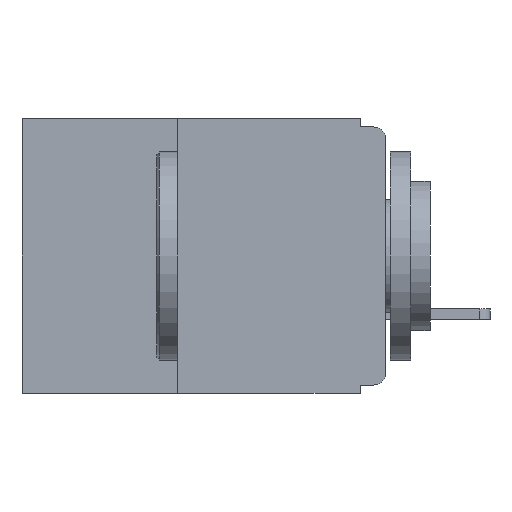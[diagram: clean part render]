
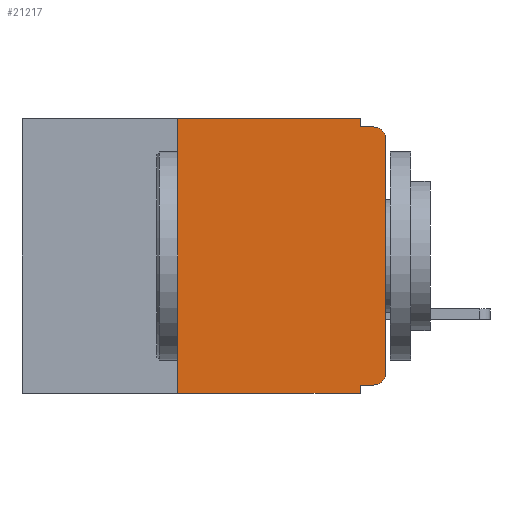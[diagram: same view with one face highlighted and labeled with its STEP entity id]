
A CAD part, left-side view. The second image highlights one B-rep face of the part: STEP entity #21217.
In plain terms, the highlighted planar face has unit normal (-1, 0, 0).
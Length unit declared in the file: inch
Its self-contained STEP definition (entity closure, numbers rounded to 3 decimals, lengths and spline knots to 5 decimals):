
#76 = ORIENTED_EDGE ( 'NONE', *, *, #14509, .T. ) ;
#262 = VERTEX_POINT ( 'NONE', #20930 ) ;
#1431 = ORIENTED_EDGE ( 'NONE', *, *, #22499, .F. ) ;
#1726 = LINE ( 'NONE', #13594, #11284 ) ;
#1873 = CARTESIAN_POINT ( 'NONE',  ( 0., 0.031, 0. ) ) ;
#2783 = CARTESIAN_POINT ( 'NONE',  ( 0., 0.031, -0.33 ) ) ;
#2972 = VERTEX_POINT ( 'NONE', #15568 ) ;
#3014 = DIRECTION ( 'NONE',  ( 1., 0., 0. ) ) ;
#3465 = CARTESIAN_POINT ( 'NONE',  ( 0., 0.437, 0. ) ) ;
#3962 = VERTEX_POINT ( 'NONE', #11965 ) ;
#4396 = DIRECTION ( 'NONE',  ( 0., 0., 1. ) ) ;
#4666 = VERTEX_POINT ( 'NONE', #12982 ) ;
#4954 = AXIS2_PLACEMENT_3D ( 'NONE', #10479, #23511, #12380 ) ;
#4986 = EDGE_CURVE ( 'NONE', #5842, #9001, #12951, .T. ) ;
#5301 = EDGE_CURVE ( 'NONE', #12902, #4666, #10860, .T. ) ;
#5350 = DIRECTION ( 'NONE',  ( 0., -1., 0. ) ) ;
#5389 = DIRECTION ( 'NONE',  ( 0., -1., 0. ) ) ;
#5541 = CARTESIAN_POINT ( 'NONE',  ( 0., 0.015, -0.305 ) ) ;
#5785 = VECTOR ( 'NONE', #5389, 39.37008 ) ;
#5842 = VERTEX_POINT ( 'NONE', #23869 ) ;
#6210 = EDGE_CURVE ( 'NONE', #6673, #262, #18990, .T. ) ;
#6287 = VECTOR ( 'NONE', #7058, 39.37008 ) ;
#6673 = VERTEX_POINT ( 'NONE', #7911 ) ;
#7019 = EDGE_CURVE ( 'NONE', #2972, #262, #21287, .T. ) ;
#7058 = DIRECTION ( 'NONE',  ( 0., -1., 0. ) ) ;
#7256 = CARTESIAN_POINT ( 'NONE',  ( 0., 0.031, 0. ) ) ;
#7468 = DIRECTION ( 'NONE',  ( 0., 0., -1. ) ) ;
#7911 = CARTESIAN_POINT ( 'NONE',  ( 0., 0.031, -0.32 ) ) ;
#8076 = CARTESIAN_POINT ( 'NONE',  ( 0., 0.015, -0.32 ) ) ;
#8418 = ORIENTED_EDGE ( 'NONE', *, *, #13133, .F. ) ;
#8632 = LINE ( 'NONE', #3465, #13662 ) ;
#9001 = VERTEX_POINT ( 'NONE', #12977 ) ;
#9172 = DIRECTION ( 'NONE',  ( 0., 0., -1. ) ) ;
#9585 = CIRCLE ( 'NONE', #4954, 0.015 ) ;
#9639 = VECTOR ( 'NONE', #16034, 39.37008 ) ;
#9664 = EDGE_CURVE ( 'NONE', #14333, #5842, #16565, .T. ) ;
#9904 = VECTOR ( 'NONE', #10613, 39.37008 ) ;
#10479 = CARTESIAN_POINT ( 'NONE',  ( 0., 0.015, -0.025 ) ) ;
#10613 = DIRECTION ( 'NONE',  ( 0., 1., 0. ) ) ;
#10860 = LINE ( 'NONE', #12954, #5785 ) ;
#11175 = ORIENTED_EDGE ( 'NONE', *, *, #6210, .F. ) ;
#11284 = VECTOR ( 'NONE', #13673, 39.37008 ) ;
#11965 = CARTESIAN_POINT ( 'NONE',  ( 0., 0.25, 0. ) ) ;
#12380 = DIRECTION ( 'NONE',  ( 0., 0., -1. ) ) ;
#12902 = VERTEX_POINT ( 'NONE', #22612 ) ;
#12951 = LINE ( 'NONE', #13851, #22836 ) ;
#12954 = CARTESIAN_POINT ( 'NONE',  ( 0., 0., -0.01 ) ) ;
#12977 = CARTESIAN_POINT ( 'NONE',  ( 0., 0., -0.025 ) ) ;
#12982 = CARTESIAN_POINT ( 'NONE',  ( 0., 0.015, -0.01 ) ) ;
#13133 = EDGE_CURVE ( 'NONE', #14333, #6673, #14932, .T. ) ;
#13594 = CARTESIAN_POINT ( 'NONE',  ( 0., 0.25, -0.33 ) ) ;
#13637 = FACE_OUTER_BOUND ( 'NONE', #20913, .T. ) ;
#13662 = VECTOR ( 'NONE', #5350, 39.37008 ) ;
#13673 = DIRECTION ( 'NONE',  ( 0., 0., 1. ) ) ;
#13851 = CARTESIAN_POINT ( 'NONE',  ( 0., 0., 0. ) ) ;
#14030 = VECTOR ( 'NONE', #9172, 39.37008 ) ;
#14333 = VERTEX_POINT ( 'NONE', #8076 ) ;
#14509 = EDGE_CURVE ( 'NONE', #9001, #4666, #9585, .T. ) ;
#14793 = VERTEX_POINT ( 'NONE', #1873 ) ;
#14805 = ORIENTED_EDGE ( 'NONE', *, *, #18618, .F. ) ;
#14932 = LINE ( 'NONE', #16227, #9904 ) ;
#15223 = AXIS2_PLACEMENT_3D ( 'NONE', #5541, #18714, #7468 ) ;
#15568 = CARTESIAN_POINT ( 'NONE',  ( 0., 0.25, -0.33 ) ) ;
#16034 = DIRECTION ( 'NONE',  ( 0., 0., -1. ) ) ;
#16227 = CARTESIAN_POINT ( 'NONE',  ( 0., 0., -0.32 ) ) ;
#16261 = DIRECTION ( 'NONE',  ( 0., 0., -1. ) ) ;
#16565 = CIRCLE ( 'NONE', #15223, 0.015 ) ;
#18161 = ORIENTED_EDGE ( 'NONE', *, *, #4986, .T. ) ;
#18618 = EDGE_CURVE ( 'NONE', #14793, #12902, #18978, .T. ) ;
#18714 = DIRECTION ( 'NONE',  ( -1., 0., 0. ) ) ;
#18978 = LINE ( 'NONE', #7256, #14030 ) ;
#18990 = LINE ( 'NONE', #2783, #9639 ) ;
#19405 = AXIS2_PLACEMENT_3D ( 'NONE', #19869, #3014, #16261 ) ;
#19869 = CARTESIAN_POINT ( 'NONE',  ( 0., 0.437, 0. ) ) ;
#20097 = ORIENTED_EDGE ( 'NONE', *, *, #20758, .F. ) ;
#20758 = EDGE_CURVE ( 'NONE', #3962, #14793, #8632, .T. ) ;
#20913 = EDGE_LOOP ( 'NONE', ( #18161, #76, #24253, #14805, #20097, #1431, #23359, #11175, #8418, #24220 ) ) ;
#20930 = CARTESIAN_POINT ( 'NONE',  ( 0., 0.031, -0.33 ) ) ;
#21217 = ADVANCED_FACE ( 'NONE', ( #13637 ), #21776, .F. ) ;
#21287 = LINE ( 'NONE', #23825, #6287 ) ;
#21776 = PLANE ( 'NONE',  #19405 ) ;
#22499 = EDGE_CURVE ( 'NONE', #2972, #3962, #1726, .T. ) ;
#22612 = CARTESIAN_POINT ( 'NONE',  ( 0., 0.031, -0.01 ) ) ;
#22836 = VECTOR ( 'NONE', #4396, 39.37008 ) ;
#23359 = ORIENTED_EDGE ( 'NONE', *, *, #7019, .T. ) ;
#23511 = DIRECTION ( 'NONE',  ( -1., 0., 0. ) ) ;
#23825 = CARTESIAN_POINT ( 'NONE',  ( 0., 0.437, -0.33 ) ) ;
#23869 = CARTESIAN_POINT ( 'NONE',  ( 0., 0., -0.305 ) ) ;
#24220 = ORIENTED_EDGE ( 'NONE', *, *, #9664, .T. ) ;
#24253 = ORIENTED_EDGE ( 'NONE', *, *, #5301, .F. ) ;
